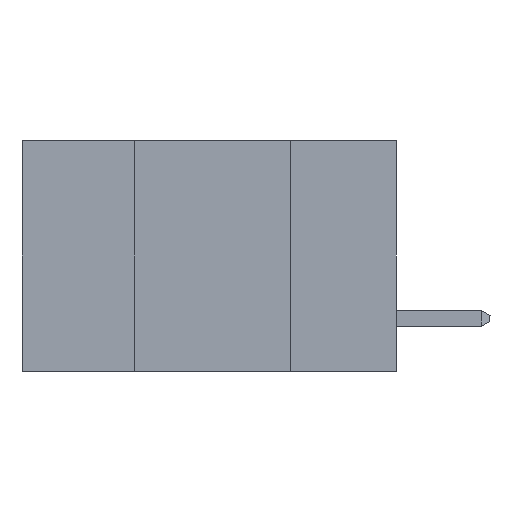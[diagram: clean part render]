
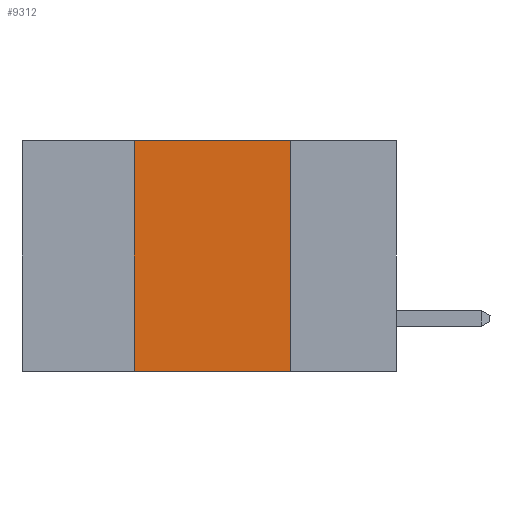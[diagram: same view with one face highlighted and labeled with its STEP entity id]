
A CAD part, left-side view. The second image highlights one B-rep face of the part: STEP entity #9312.
In plain terms, the highlighted planar face has unit normal (-1, 0, 0).
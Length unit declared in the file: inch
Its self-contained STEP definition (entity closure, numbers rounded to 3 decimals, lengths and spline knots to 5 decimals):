
#836 = EDGE_CURVE ( 'NONE', #8484, #6482, #6080, .T. ) ;
#959 = DIRECTION ( 'NONE',  ( 0., 0., 1. ) ) ;
#1717 = CARTESIAN_POINT ( 'NONE',  ( 0., 0.17, -0.37 ) ) ;
#1947 = EDGE_CURVE ( 'NONE', #5047, #8484, #6657, .T. ) ;
#1996 = EDGE_LOOP ( 'NONE', ( #9181, #10070, #8059, #9998 ) ) ;
#2718 = CARTESIAN_POINT ( 'NONE',  ( 0., 0.42, 0. ) ) ;
#3092 = DIRECTION ( 'NONE',  ( 1., 0., 0. ) ) ;
#3153 = PLANE ( 'NONE',  #9628 ) ;
#3284 = CARTESIAN_POINT ( 'NONE',  ( 0., 0.17, 0. ) ) ;
#3872 = FACE_OUTER_BOUND ( 'NONE', #1996, .T. ) ;
#4478 = CARTESIAN_POINT ( 'NONE',  ( 0., 0.17, -0.37 ) ) ;
#4883 = CARTESIAN_POINT ( 'NONE',  ( 0., 0.6, 0. ) ) ;
#4969 = DIRECTION ( 'NONE',  ( 0., -1., 0. ) ) ;
#5047 = VERTEX_POINT ( 'NONE', #2718 ) ;
#5413 = CARTESIAN_POINT ( 'NONE',  ( 0., 0.42, -0.37 ) ) ;
#5474 = VECTOR ( 'NONE', #4969, 39.37008 ) ;
#5654 = DIRECTION ( 'NONE',  ( 0., 0., -1. ) ) ;
#5838 = DIRECTION ( 'NONE',  ( 0., -1., 0. ) ) ;
#5884 = EDGE_CURVE ( 'NONE', #10654, #6482, #9137, .T. ) ;
#5956 = EDGE_CURVE ( 'NONE', #10654, #5047, #8695, .T. ) ;
#6080 = LINE ( 'NONE', #4478, #7648 ) ;
#6209 = CARTESIAN_POINT ( 'NONE',  ( 0., 0.42, -0.37 ) ) ;
#6482 = VERTEX_POINT ( 'NONE', #1717 ) ;
#6657 = LINE ( 'NONE', #10772, #10069 ) ;
#7601 = CARTESIAN_POINT ( 'NONE',  ( 0., 0.6, -0.37 ) ) ;
#7648 = VECTOR ( 'NONE', #10418, 39.37008 ) ;
#8059 = ORIENTED_EDGE ( 'NONE', *, *, #5956, .F. ) ;
#8484 = VERTEX_POINT ( 'NONE', #3284 ) ;
#8695 = LINE ( 'NONE', #6209, #10201 ) ;
#9137 = LINE ( 'NONE', #7601, #5474 ) ;
#9181 = ORIENTED_EDGE ( 'NONE', *, *, #836, .F. ) ;
#9312 = ADVANCED_FACE ( 'NONE', ( #3872 ), #3153, .F. ) ;
#9628 = AXIS2_PLACEMENT_3D ( 'NONE', #4883, #3092, #5654 ) ;
#9998 = ORIENTED_EDGE ( 'NONE', *, *, #5884, .T. ) ;
#10069 = VECTOR ( 'NONE', #5838, 39.37008 ) ;
#10070 = ORIENTED_EDGE ( 'NONE', *, *, #1947, .F. ) ;
#10201 = VECTOR ( 'NONE', #959, 39.37008 ) ;
#10418 = DIRECTION ( 'NONE',  ( 0., 0., -1. ) ) ;
#10654 = VERTEX_POINT ( 'NONE', #5413 ) ;
#10772 = CARTESIAN_POINT ( 'NONE',  ( 0., 0.6, 0. ) ) ;
